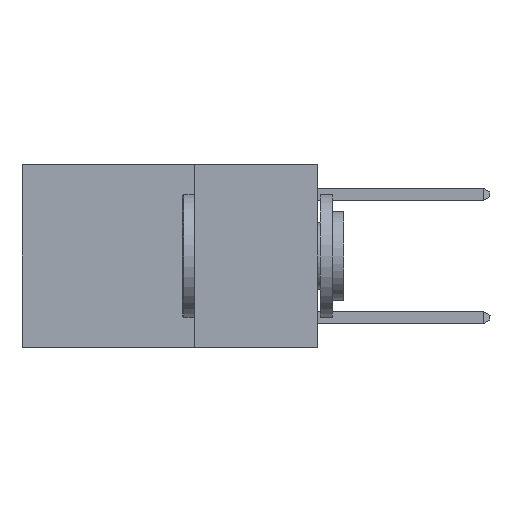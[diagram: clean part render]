
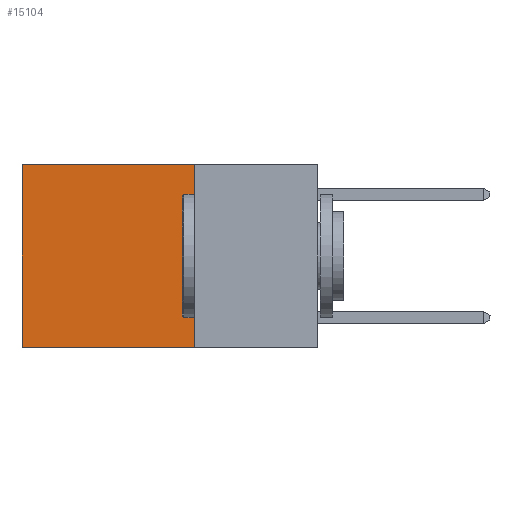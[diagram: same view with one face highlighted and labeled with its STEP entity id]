
A CAD part, left-side view. The second image highlights one B-rep face of the part: STEP entity #15104.
In plain terms, the highlighted planar face has unit normal (-1, 0, 0).
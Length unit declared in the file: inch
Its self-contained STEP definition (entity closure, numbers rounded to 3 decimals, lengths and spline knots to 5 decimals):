
#634 = DIRECTION ( 'NONE',  ( 0., 0., -1. ) ) ;
#1270 = CARTESIAN_POINT ( 'NONE',  ( 0.2625, 0.25, 0. ) ) ;
#2776 = EDGE_LOOP ( 'NONE', ( #12069, #5052, #15099, #12695 ) ) ;
#3152 = AXIS2_PLACEMENT_3D ( 'NONE', #11859, #4617, #14629 ) ;
#3296 = EDGE_CURVE ( 'NONE', #17934, #14317, #8639, .T. ) ;
#3453 = CARTESIAN_POINT ( 'NONE',  ( 0.2625, 0.25, -0.37 ) ) ;
#3822 = CARTESIAN_POINT ( 'NONE',  ( 0.2625, 0.6, 0. ) ) ;
#4081 = EDGE_CURVE ( 'NONE', #17943, #6023, #11754, .T. ) ;
#4617 = DIRECTION ( 'NONE',  ( 1., 0., 0. ) ) ;
#5052 = ORIENTED_EDGE ( 'NONE', *, *, #14510, .F. ) ;
#6023 = VERTEX_POINT ( 'NONE', #9303 ) ;
#7515 = PLANE ( 'NONE',  #3152 ) ;
#7926 = VECTOR ( 'NONE', #11516, 39.37008 ) ;
#8639 = LINE ( 'NONE', #17646, #12447 ) ;
#9303 = CARTESIAN_POINT ( 'NONE',  ( 0.2625, 0.25, -0.37 ) ) ;
#9713 = CARTESIAN_POINT ( 'NONE',  ( 0.2625, 0.25, 0. ) ) ;
#9793 = LINE ( 'NONE', #11003, #16308 ) ;
#10058 = FACE_OUTER_BOUND ( 'NONE', #2776, .T. ) ;
#11003 = CARTESIAN_POINT ( 'NONE',  ( 0.2625, 0.25, 0. ) ) ;
#11516 = DIRECTION ( 'NONE',  ( 0., 0., -1. ) ) ;
#11754 = LINE ( 'NONE', #1270, #7926 ) ;
#11859 = CARTESIAN_POINT ( 'NONE',  ( 0.2625, 0.25, 0. ) ) ;
#12069 = ORIENTED_EDGE ( 'NONE', *, *, #3296, .T. ) ;
#12187 = DIRECTION ( 'NONE',  ( 0., 1., 0. ) ) ;
#12408 = DIRECTION ( 'NONE',  ( 0., 1., 0. ) ) ;
#12447 = VECTOR ( 'NONE', #634, 39.37008 ) ;
#12695 = ORIENTED_EDGE ( 'NONE', *, *, #17822, .T. ) ;
#13859 = VECTOR ( 'NONE', #12187, 39.37008 ) ;
#14317 = VERTEX_POINT ( 'NONE', #15882 ) ;
#14510 = EDGE_CURVE ( 'NONE', #6023, #14317, #17773, .T. ) ;
#14629 = DIRECTION ( 'NONE',  ( 0., 0., -1. ) ) ;
#15099 = ORIENTED_EDGE ( 'NONE', *, *, #4081, .F. ) ;
#15104 = ADVANCED_FACE ( 'NONE', ( #10058 ), #7515, .F. ) ;
#15882 = CARTESIAN_POINT ( 'NONE',  ( 0.2625, 0.6, -0.37 ) ) ;
#16308 = VECTOR ( 'NONE', #12408, 39.37008 ) ;
#17646 = CARTESIAN_POINT ( 'NONE',  ( 0.2625, 0.6, 0. ) ) ;
#17773 = LINE ( 'NONE', #3453, #13859 ) ;
#17822 = EDGE_CURVE ( 'NONE', #17943, #17934, #9793, .T. ) ;
#17934 = VERTEX_POINT ( 'NONE', #3822 ) ;
#17943 = VERTEX_POINT ( 'NONE', #9713 ) ;
